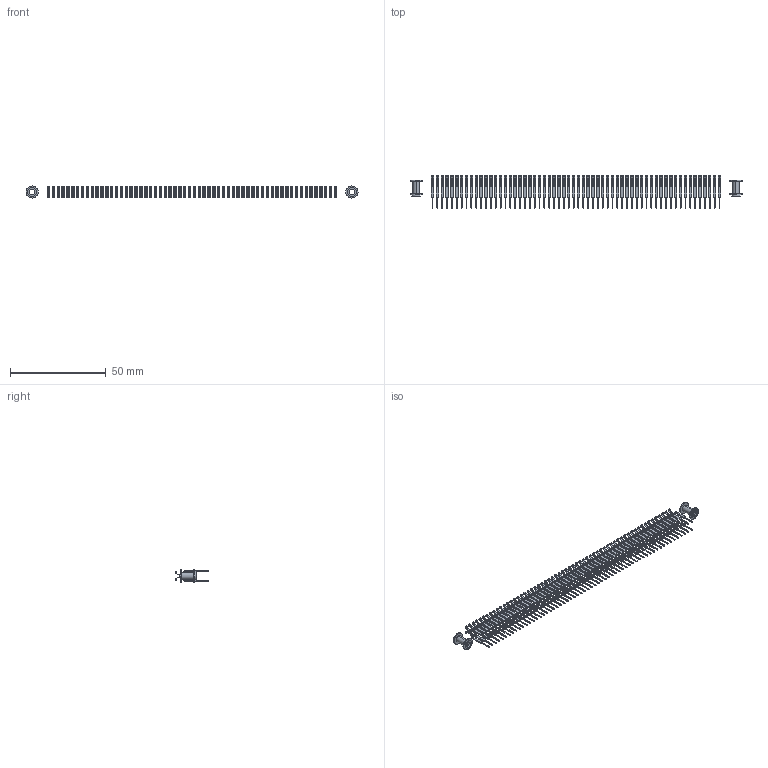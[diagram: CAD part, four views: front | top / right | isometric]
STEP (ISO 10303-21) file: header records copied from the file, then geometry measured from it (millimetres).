
FILE_DESCRIPTION (( 'STEP AP203' ), '1' );
FILE_NAME ('345-120-525-803.STEP', '2020-09-22T00:48:27', ( '' ), ( '' ), 'SwSTEP 2.0', 'SolidWorks 2020', '' );
FILE_SCHEMA (( 'CONFIG_CONTROL_DESIGN' ));
Length unit declared in the file: inch
Products named in the file (4): 345 Part_0.170 Offset - 0.156 Dia-TH; 345-250-002_345-250-002-102; 345-292-001_345-293-125; 345-120-525-803
Assembly tree (123 placements, depth 2):
  345-120-525-803
    345 Part_0.170 Offset - 0.156 Dia-TH
    345-292-001_345-293-125  x120
    345-250-002_345-250-002-102  x2
Bounding box: 173.35 x 17.14 x 6.35 mm (x, y, z)
Volume: 991.4 mm3; surface area: 7386.5 mm2
Topology: 122 solids, 122 shells, 5558 faces, 15196 edges, 9648 vertices
Faces by surface type: plane 3850, cylinder 1700, cone 8
Entity records: 45510 total; most frequent: CARTESIAN_POINT 7587, ORIENTED_EDGE 7514, DIRECTION 6699, EDGE_CURVE 3757, VECTOR 3365, LINE 3365, VERTEX_POINT 2498, AXIS2_PLACEMENT_3D 1667
